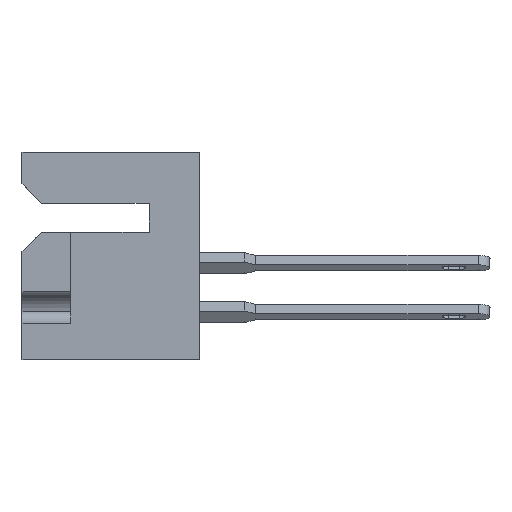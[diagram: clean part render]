
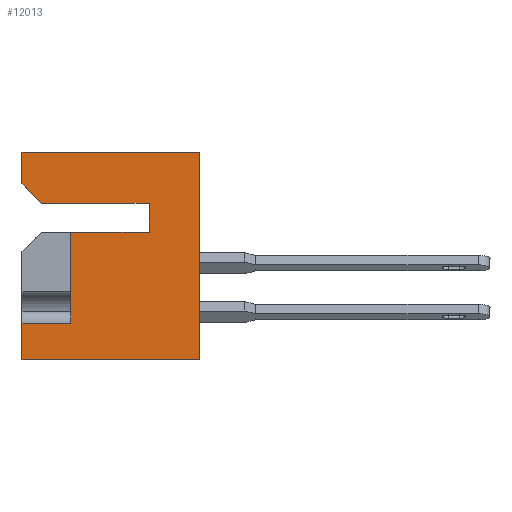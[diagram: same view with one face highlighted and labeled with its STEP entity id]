
A CAD part, left-side view. The second image highlights one B-rep face of the part: STEP entity #12013.
In plain terms, the highlighted planar face has unit normal (-1, 0, 0).
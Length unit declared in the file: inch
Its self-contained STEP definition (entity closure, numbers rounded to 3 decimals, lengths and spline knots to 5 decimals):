
#569 = EDGE_CURVE ( 'NONE', #3936, #2068, #8911, .T. ) ;
#1052 = ORIENTED_EDGE ( 'NONE', *, *, #17506, .T. ) ;
#1340 = VERTEX_POINT ( 'NONE', #1728 ) ;
#1529 = VERTEX_POINT ( 'NONE', #18251 ) ;
#1728 = CARTESIAN_POINT ( 'NONE',  ( 0., 0.453, -0.081 ) ) ;
#2068 = VERTEX_POINT ( 'NONE', #11704 ) ;
#2533 = CARTESIAN_POINT ( 'NONE',  ( 0., 0.453, -0.531 ) ) ;
#2783 = VECTOR ( 'NONE', #11434, 39.37008 ) ;
#2873 = CARTESIAN_POINT ( 'NONE',  ( 0., 0.328, -0.205 ) ) ;
#2925 = EDGE_CURVE ( 'NONE', #1340, #1529, #7677, .T. ) ;
#3163 = DIRECTION ( 'NONE',  ( 0., -0.707, -0.707 ) ) ;
#3167 = DIRECTION ( 'NONE',  ( 0., 0., 1. ) ) ;
#3264 = LINE ( 'NONE', #12941, #2783 ) ;
#3584 = ORIENTED_EDGE ( 'NONE', *, *, #20185, .F. ) ;
#3685 = EDGE_CURVE ( 'NONE', #1340, #19631, #10474, .T. ) ;
#3724 = FACE_OUTER_BOUND ( 'NONE', #6132, .T. ) ;
#3936 = VERTEX_POINT ( 'NONE', #2533 ) ;
#4161 = DIRECTION ( 'NONE',  ( 1., 0., 0. ) ) ;
#4170 = ORIENTED_EDGE ( 'NONE', *, *, #19253, .F. ) ;
#4311 = DIRECTION ( 'NONE',  ( 0., 0., 1. ) ) ;
#4498 = ORIENTED_EDGE ( 'NONE', *, *, #14633, .F. ) ;
#4580 = CARTESIAN_POINT ( 'NONE',  ( 0., 0.453, 0. ) ) ;
#5143 = VERTEX_POINT ( 'NONE', #2873 ) ;
#5422 = ORIENTED_EDGE ( 'NONE', *, *, #569, .T. ) ;
#5484 = VECTOR ( 'NONE', #3167, 39.37008 ) ;
#5560 = CARTESIAN_POINT ( 'NONE',  ( 0., 0.403, -0.131 ) ) ;
#5568 = EDGE_CURVE ( 'NONE', #1529, #12908, #20913, .T. ) ;
#5618 = DIRECTION ( 'NONE',  ( 0., -1., 0. ) ) ;
#6018 = DIRECTION ( 'NONE',  ( 0., 1., 0. ) ) ;
#6105 = AXIS2_PLACEMENT_3D ( 'NONE', #7245, #4161, #8935 ) ;
#6132 = EDGE_LOOP ( 'NONE', ( #1052, #3584, #5422, #7942, #13577, #13890, #8461, #4170, #10184, #7049, #4498 ) ) ;
#6481 = EDGE_CURVE ( 'NONE', #2068, #12908, #3264, .T. ) ;
#6726 = LINE ( 'NONE', #11769, #15653 ) ;
#6876 = CARTESIAN_POINT ( 'NONE',  ( 0., 0.453, -0.531 ) ) ;
#7049 = ORIENTED_EDGE ( 'NONE', *, *, #13938, .T. ) ;
#7245 = CARTESIAN_POINT ( 'NONE',  ( 0., 0.453, 0. ) ) ;
#7677 = LINE ( 'NONE', #4580, #17353 ) ;
#7698 = VERTEX_POINT ( 'NONE', #9502 ) ;
#7748 = CARTESIAN_POINT ( 'NONE',  ( 0., 0.403, -0.131 ) ) ;
#7942 = ORIENTED_EDGE ( 'NONE', *, *, #6481, .T. ) ;
#8461 = ORIENTED_EDGE ( 'NONE', *, *, #3685, .T. ) ;
#8604 = VERTEX_POINT ( 'NONE', #12069 ) ;
#8911 = LINE ( 'NONE', #6876, #10962 ) ;
#8935 = DIRECTION ( 'NONE',  ( 0., 0., -1. ) ) ;
#9502 = CARTESIAN_POINT ( 'NONE',  ( 0., 0.453, -0.437 ) ) ;
#9811 = CARTESIAN_POINT ( 'NONE',  ( 0., 0., 0. ) ) ;
#10048 = CARTESIAN_POINT ( 'NONE',  ( 0., 0.453, 0. ) ) ;
#10162 = CARTESIAN_POINT ( 'NONE',  ( 0., 0.328, -0.437 ) ) ;
#10184 = ORIENTED_EDGE ( 'NONE', *, *, #17230, .F. ) ;
#10474 = LINE ( 'NONE', #7748, #11216 ) ;
#10515 = CARTESIAN_POINT ( 'NONE',  ( 0., 0.328, -0.437 ) ) ;
#10946 = CARTESIAN_POINT ( 'NONE',  ( 0., 0.128, -0.131 ) ) ;
#10962 = VECTOR ( 'NONE', #18247, 39.37008 ) ;
#11216 = VECTOR ( 'NONE', #3163, 39.37008 ) ;
#11434 = DIRECTION ( 'NONE',  ( 0., 0., 1. ) ) ;
#11704 = CARTESIAN_POINT ( 'NONE',  ( 0., 0., -0.531 ) ) ;
#11769 = CARTESIAN_POINT ( 'NONE',  ( 0., 0.128, -0.205 ) ) ;
#12013 = ADVANCED_FACE ( 'NONE', ( #3724 ), #15482, .F. ) ;
#12069 = CARTESIAN_POINT ( 'NONE',  ( 0., 0.128, -0.205 ) ) ;
#12144 = VECTOR ( 'NONE', #15072, 39.37008 ) ;
#12275 = VECTOR ( 'NONE', #16713, 39.37008 ) ;
#12898 = LINE ( 'NONE', #10162, #12144 ) ;
#12908 = VERTEX_POINT ( 'NONE', #9811 ) ;
#12941 = CARTESIAN_POINT ( 'NONE',  ( 0., 0., 0. ) ) ;
#12955 = CARTESIAN_POINT ( 'NONE',  ( 0., 0.128, -0.131 ) ) ;
#13272 = LINE ( 'NONE', #10048, #12275 ) ;
#13303 = VECTOR ( 'NONE', #5618, 39.37008 ) ;
#13577 = ORIENTED_EDGE ( 'NONE', *, *, #5568, .F. ) ;
#13890 = ORIENTED_EDGE ( 'NONE', *, *, #2925, .F. ) ;
#13938 = EDGE_CURVE ( 'NONE', #8604, #5143, #6726, .T. ) ;
#14287 = CARTESIAN_POINT ( 'NONE',  ( 0., 0.128, -0.131 ) ) ;
#14339 = VECTOR ( 'NONE', #17953, 39.37008 ) ;
#14633 = EDGE_CURVE ( 'NONE', #18173, #5143, #15609, .T. ) ;
#15072 = DIRECTION ( 'NONE',  ( 0., 1., 0. ) ) ;
#15391 = CARTESIAN_POINT ( 'NONE',  ( 0., 0.453, 0. ) ) ;
#15482 = PLANE ( 'NONE',  #6105 ) ;
#15609 = LINE ( 'NONE', #17886, #14339 ) ;
#15653 = VECTOR ( 'NONE', #18152, 39.37008 ) ;
#15846 = VECTOR ( 'NONE', #6018, 39.37008 ) ;
#16350 = LINE ( 'NONE', #10946, #15846 ) ;
#16713 = DIRECTION ( 'NONE',  ( 0., 0., 1. ) ) ;
#17230 = EDGE_CURVE ( 'NONE', #8604, #17574, #20018, .T. ) ;
#17353 = VECTOR ( 'NONE', #4311, 39.37008 ) ;
#17506 = EDGE_CURVE ( 'NONE', #18173, #7698, #12898, .T. ) ;
#17574 = VERTEX_POINT ( 'NONE', #14287 ) ;
#17886 = CARTESIAN_POINT ( 'NONE',  ( 0., 0.328, -0.205 ) ) ;
#17953 = DIRECTION ( 'NONE',  ( 0., 0., 1. ) ) ;
#18152 = DIRECTION ( 'NONE',  ( 0., 1., 0. ) ) ;
#18173 = VERTEX_POINT ( 'NONE', #10515 ) ;
#18247 = DIRECTION ( 'NONE',  ( 0., -1., 0. ) ) ;
#18251 = CARTESIAN_POINT ( 'NONE',  ( 0., 0.453, 0. ) ) ;
#19253 = EDGE_CURVE ( 'NONE', #17574, #19631, #16350, .T. ) ;
#19631 = VERTEX_POINT ( 'NONE', #5560 ) ;
#20018 = LINE ( 'NONE', #12955, #5484 ) ;
#20185 = EDGE_CURVE ( 'NONE', #3936, #7698, #13272, .T. ) ;
#20913 = LINE ( 'NONE', #15391, #13303 ) ;
